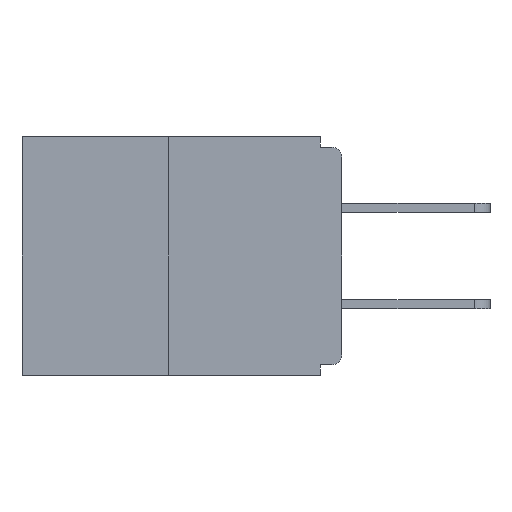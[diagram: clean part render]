
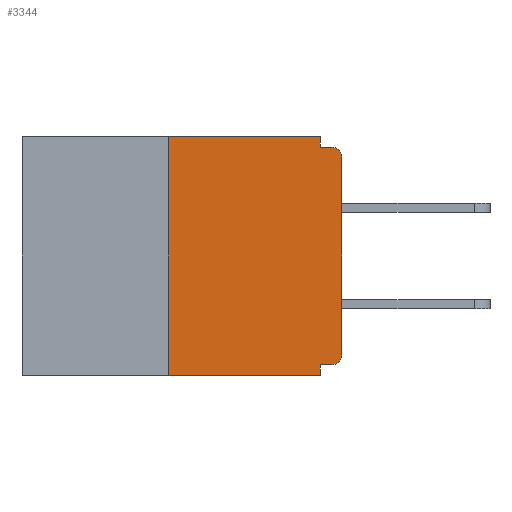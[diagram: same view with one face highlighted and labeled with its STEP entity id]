
A CAD part, left-side view. The second image highlights one B-rep face of the part: STEP entity #3344.
In plain terms, the highlighted planar face has unit normal (-1, 0, 0).
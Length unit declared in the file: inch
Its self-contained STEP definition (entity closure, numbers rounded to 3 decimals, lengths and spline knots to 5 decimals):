
#42 = VERTEX_POINT ( 'NONE', #8727 ) ;
#74 = DIRECTION ( 'NONE',  ( 0., 0., -1. ) ) ;
#261 = ORIENTED_EDGE ( 'NONE', *, *, #8224, .T. ) ;
#411 = LINE ( 'NONE', #10437, #16198 ) ;
#817 = ORIENTED_EDGE ( 'NONE', *, *, #2621, .T. ) ;
#1065 = AXIS2_PLACEMENT_3D ( 'NONE', #19372, #4095, #16201 ) ;
#1388 = VECTOR ( 'NONE', #17654, 39.37008 ) ;
#1425 = CARTESIAN_POINT ( 'NONE',  ( 0., 0.031, 0. ) ) ;
#1611 = ORIENTED_EDGE ( 'NONE', *, *, #13502, .T. ) ;
#1854 = VECTOR ( 'NONE', #16144, 39.37008 ) ;
#1943 = DIRECTION ( 'NONE',  ( 0., 0., 1. ) ) ;
#1983 = EDGE_CURVE ( 'NONE', #3503, #18211, #15002, .T. ) ;
#2029 = VECTOR ( 'NONE', #1943, 39.37008 ) ;
#2291 = FACE_OUTER_BOUND ( 'NONE', #15684, .T. ) ;
#2348 = AXIS2_PLACEMENT_3D ( 'NONE', #12763, #17445, #6709 ) ;
#2370 = EDGE_CURVE ( 'NONE', #18449, #11991, #411, .T. ) ;
#2621 = EDGE_CURVE ( 'NONE', #12893, #10012, #4950, .T. ) ;
#2748 = VECTOR ( 'NONE', #10652, 39.37008 ) ;
#2923 = CARTESIAN_POINT ( 'NONE',  ( 0., 0.031, -0.343 ) ) ;
#3344 = ADVANCED_FACE ( 'NONE', ( #2291 ), #6649, .F. ) ;
#3503 = VERTEX_POINT ( 'NONE', #7133 ) ;
#3613 = VERTEX_POINT ( 'NONE', #15582 ) ;
#3768 = LINE ( 'NONE', #1425, #5700 ) ;
#4095 = DIRECTION ( 'NONE',  ( -1., 0., 0. ) ) ;
#4348 = CARTESIAN_POINT ( 'NONE',  ( 0., 0.25, -0.343 ) ) ;
#4840 = CARTESIAN_POINT ( 'NONE',  ( 0., 0., -0.03 ) ) ;
#4950 = CIRCLE ( 'NONE', #1065, 0.015 ) ;
#5155 = EDGE_CURVE ( 'NONE', #42, #10012, #15229, .T. ) ;
#5700 = VECTOR ( 'NONE', #74, 39.37008 ) ;
#6503 = ORIENTED_EDGE ( 'NONE', *, *, #17656, .T. ) ;
#6649 = PLANE ( 'NONE',  #2348 ) ;
#6709 = DIRECTION ( 'NONE',  ( 0., 0., -1. ) ) ;
#6756 = EDGE_CURVE ( 'NONE', #7740, #18449, #18314, .T. ) ;
#6788 = ORIENTED_EDGE ( 'NONE', *, *, #13389, .F. ) ;
#7002 = EDGE_CURVE ( 'NONE', #18211, #3613, #15166, .T. ) ;
#7036 = CIRCLE ( 'NONE', #7235, 0.015 ) ;
#7133 = CARTESIAN_POINT ( 'NONE',  ( 0., 0.015, -0.328 ) ) ;
#7235 = AXIS2_PLACEMENT_3D ( 'NONE', #13138, #9988, #19256 ) ;
#7285 = DIRECTION ( 'NONE',  ( 0., -1., 0. ) ) ;
#7740 = VERTEX_POINT ( 'NONE', #4348 ) ;
#7878 = VERTEX_POINT ( 'NONE', #13826 ) ;
#8224 = EDGE_CURVE ( 'NONE', #3503, #7878, #7036, .T. ) ;
#8343 = CARTESIAN_POINT ( 'NONE',  ( 0., 0.015, -0.015 ) ) ;
#8727 = CARTESIAN_POINT ( 'NONE',  ( 0., 0.031, -0.015 ) ) ;
#9315 = ORIENTED_EDGE ( 'NONE', *, *, #2370, .F. ) ;
#9682 = LINE ( 'NONE', #14432, #15375 ) ;
#9988 = DIRECTION ( 'NONE',  ( -1., 0., 0. ) ) ;
#10012 = VERTEX_POINT ( 'NONE', #8343 ) ;
#10437 = CARTESIAN_POINT ( 'NONE',  ( 0., 0.46, 0. ) ) ;
#10652 = DIRECTION ( 'NONE',  ( 0., 0., -1. ) ) ;
#11117 = CARTESIAN_POINT ( 'NONE',  ( 0., 0.25, 0. ) ) ;
#11199 = CARTESIAN_POINT ( 'NONE',  ( 0., 0.031, -0.328 ) ) ;
#11991 = VERTEX_POINT ( 'NONE', #16239 ) ;
#12010 = ORIENTED_EDGE ( 'NONE', *, *, #1983, .F. ) ;
#12066 = ORIENTED_EDGE ( 'NONE', *, *, #7002, .F. ) ;
#12396 = CARTESIAN_POINT ( 'NONE',  ( 0., 0.46, -0.343 ) ) ;
#12763 = CARTESIAN_POINT ( 'NONE',  ( 0., 0.46, 0. ) ) ;
#12893 = VERTEX_POINT ( 'NONE', #4840 ) ;
#13138 = CARTESIAN_POINT ( 'NONE',  ( 0., 0.015, -0.313 ) ) ;
#13309 = CARTESIAN_POINT ( 'NONE',  ( 0., 0., -0.015 ) ) ;
#13389 = EDGE_CURVE ( 'NONE', #11991, #42, #3768, .T. ) ;
#13502 = EDGE_CURVE ( 'NONE', #7740, #3613, #19792, .T. ) ;
#13826 = CARTESIAN_POINT ( 'NONE',  ( 0., 0., -0.313 ) ) ;
#14036 = VECTOR ( 'NONE', #14773, 39.37008 ) ;
#14243 = ORIENTED_EDGE ( 'NONE', *, *, #5155, .F. ) ;
#14432 = CARTESIAN_POINT ( 'NONE',  ( 0., 0., 0. ) ) ;
#14773 = DIRECTION ( 'NONE',  ( 0., -1., 0. ) ) ;
#15002 = LINE ( 'NONE', #15777, #1388 ) ;
#15166 = LINE ( 'NONE', #2923, #2748 ) ;
#15229 = LINE ( 'NONE', #13309, #14036 ) ;
#15375 = VECTOR ( 'NONE', #16048, 39.37008 ) ;
#15582 = CARTESIAN_POINT ( 'NONE',  ( 0., 0.031, -0.343 ) ) ;
#15684 = EDGE_LOOP ( 'NONE', ( #9315, #18428, #1611, #12066, #12010, #261, #6503, #817, #14243, #6788 ) ) ;
#15777 = CARTESIAN_POINT ( 'NONE',  ( 0., 0., -0.328 ) ) ;
#16048 = DIRECTION ( 'NONE',  ( 0., 0., 1. ) ) ;
#16144 = DIRECTION ( 'NONE',  ( 0., -1., 0. ) ) ;
#16198 = VECTOR ( 'NONE', #7285, 39.37008 ) ;
#16201 = DIRECTION ( 'NONE',  ( 0., 0., -1. ) ) ;
#16239 = CARTESIAN_POINT ( 'NONE',  ( 0., 0.031, 0. ) ) ;
#16350 = CARTESIAN_POINT ( 'NONE',  ( 0., 0.25, 0. ) ) ;
#17445 = DIRECTION ( 'NONE',  ( 1., 0., 0. ) ) ;
#17654 = DIRECTION ( 'NONE',  ( 0., 1., 0. ) ) ;
#17656 = EDGE_CURVE ( 'NONE', #7878, #12893, #9682, .T. ) ;
#18211 = VERTEX_POINT ( 'NONE', #11199 ) ;
#18314 = LINE ( 'NONE', #11117, #2029 ) ;
#18428 = ORIENTED_EDGE ( 'NONE', *, *, #6756, .F. ) ;
#18449 = VERTEX_POINT ( 'NONE', #16350 ) ;
#19256 = DIRECTION ( 'NONE',  ( 0., 0., -1. ) ) ;
#19372 = CARTESIAN_POINT ( 'NONE',  ( 0., 0.015, -0.03 ) ) ;
#19792 = LINE ( 'NONE', #12396, #1854 ) ;
